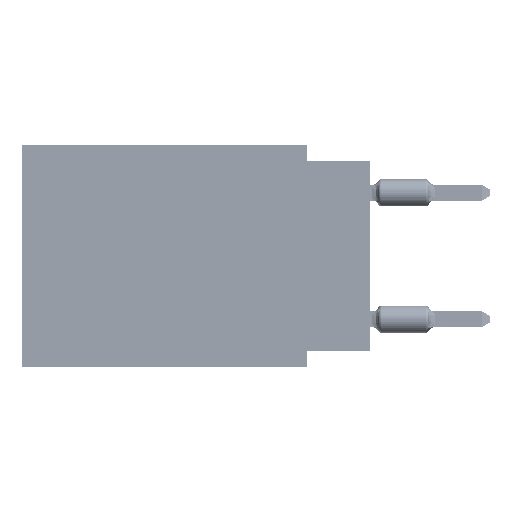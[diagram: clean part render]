
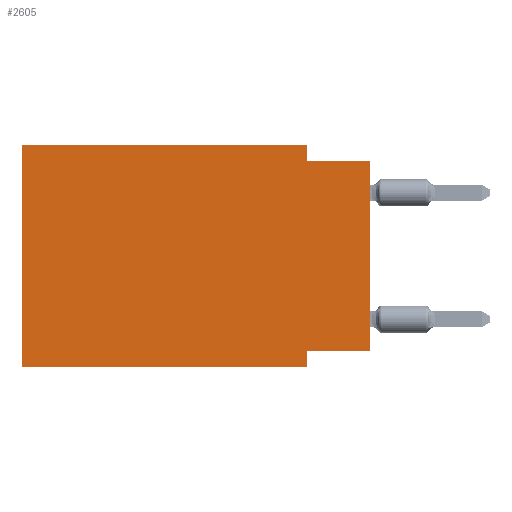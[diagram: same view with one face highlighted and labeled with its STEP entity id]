
A CAD part, left-side view. The second image highlights one B-rep face of the part: STEP entity #2605.
In plain terms, the highlighted planar face has unit normal (-1, 0, 0).
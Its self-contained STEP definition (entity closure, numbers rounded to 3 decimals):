
#426 = LINE ( 'NONE', #57246, #10804 ) ;
#1411 = ORIENTED_EDGE ( 'NONE', *, *, #46097, .F. ) ;
#2605 = ADVANCED_FACE ( 'NONE', ( #30433 ), #25722, .F. ) ;
#3043 = EDGE_CURVE ( 'NONE', #26202, #23078, #17483, .T. ) ;
#6856 = EDGE_CURVE ( 'NONE', #44678, #13129, #14527, .T. ) ;
#10655 = LINE ( 'NONE', #24699, #14334 ) ;
#10804 = VECTOR ( 'NONE', #43178, 1000. ) ;
#12487 = DIRECTION ( 'NONE',  ( 0., -1., 0. ) ) ;
#12929 = LINE ( 'NONE', #26066, #41188 ) ;
#13129 = VERTEX_POINT ( 'NONE', #49657 ) ;
#14241 = CARTESIAN_POINT ( 'NONE',  ( 0., 2.54, -0.635 ) ) ;
#14334 = VECTOR ( 'NONE', #34679, 1000. ) ;
#14527 = LINE ( 'NONE', #56056, #20309 ) ;
#17483 = LINE ( 'NONE', #32137, #44723 ) ;
#18924 = CARTESIAN_POINT ( 'NONE',  ( 0., 13.97, 0. ) ) ;
#20309 = VECTOR ( 'NONE', #41982, 1000. ) ;
#20555 = CARTESIAN_POINT ( 'NONE',  ( 0., 2.54, -8.89 ) ) ;
#22082 = VECTOR ( 'NONE', #31061, 1000. ) ;
#23078 = VERTEX_POINT ( 'NONE', #20555 ) ;
#23688 = EDGE_CURVE ( 'NONE', #13129, #52349, #59477, .T. ) ;
#24699 = CARTESIAN_POINT ( 'NONE',  ( 0., 0., 0. ) ) ;
#24920 = CARTESIAN_POINT ( 'NONE',  ( 0., 13.97, 0. ) ) ;
#25722 = PLANE ( 'NONE',  #50125 ) ;
#26066 = CARTESIAN_POINT ( 'NONE',  ( 0., 2.54, -8.89 ) ) ;
#26202 = VERTEX_POINT ( 'NONE', #37062 ) ;
#27254 = VECTOR ( 'NONE', #61697, 1000. ) ;
#28068 = LINE ( 'NONE', #52106, #59864 ) ;
#28915 = LINE ( 'NONE', #18924, #27254 ) ;
#29995 = EDGE_CURVE ( 'NONE', #55369, #46451, #10655, .T. ) ;
#30433 = FACE_OUTER_BOUND ( 'NONE', #59432, .T. ) ;
#31061 = DIRECTION ( 'NONE',  ( 0., 0., -1. ) ) ;
#32137 = CARTESIAN_POINT ( 'NONE',  ( 0., 13.97, -8.89 ) ) ;
#32706 = ORIENTED_EDGE ( 'NONE', *, *, #44882, .F. ) ;
#32989 = VERTEX_POINT ( 'NONE', #52696 ) ;
#34679 = DIRECTION ( 'NONE',  ( 0., 0., 1. ) ) ;
#35048 = CARTESIAN_POINT ( 'NONE',  ( 0., 0., -8.255 ) ) ;
#35105 = DIRECTION ( 'NONE',  ( 0., 0., -1. ) ) ;
#37062 = CARTESIAN_POINT ( 'NONE',  ( 0., 13.97, -8.89 ) ) ;
#37529 = ORIENTED_EDGE ( 'NONE', *, *, #6856, .F. ) ;
#37694 = ORIENTED_EDGE ( 'NONE', *, *, #55129, .F. ) ;
#40541 = ORIENTED_EDGE ( 'NONE', *, *, #23688, .F. ) ;
#41188 = VECTOR ( 'NONE', #45103, 1000. ) ;
#41982 = DIRECTION ( 'NONE',  ( 0., -1., 0. ) ) ;
#42424 = DIRECTION ( 'NONE',  ( 0., -1., 0. ) ) ;
#43178 = DIRECTION ( 'NONE',  ( 0., 1., 0. ) ) ;
#43928 = EDGE_CURVE ( 'NONE', #32989, #23078, #12929, .T. ) ;
#44156 = ORIENTED_EDGE ( 'NONE', *, *, #29995, .T. ) ;
#44678 = VERTEX_POINT ( 'NONE', #24920 ) ;
#44723 = VECTOR ( 'NONE', #12487, 1000. ) ;
#44882 = EDGE_CURVE ( 'NONE', #26202, #44678, #28915, .T. ) ;
#45103 = DIRECTION ( 'NONE',  ( 0., 0., -1. ) ) ;
#46097 = EDGE_CURVE ( 'NONE', #52349, #46451, #28068, .T. ) ;
#46451 = VERTEX_POINT ( 'NONE', #47879 ) ;
#47879 = CARTESIAN_POINT ( 'NONE',  ( 0., 0., -0.635 ) ) ;
#49154 = CARTESIAN_POINT ( 'NONE',  ( 0., 13.97, 0. ) ) ;
#49657 = CARTESIAN_POINT ( 'NONE',  ( 0., 2.54, 0. ) ) ;
#50125 = AXIS2_PLACEMENT_3D ( 'NONE', #49154, #54450, #35105 ) ;
#50896 = ORIENTED_EDGE ( 'NONE', *, *, #3043, .T. ) ;
#51017 = CARTESIAN_POINT ( 'NONE',  ( 0., 2.54, 0. ) ) ;
#52106 = CARTESIAN_POINT ( 'NONE',  ( 0., 0., -0.635 ) ) ;
#52349 = VERTEX_POINT ( 'NONE', #14241 ) ;
#52696 = CARTESIAN_POINT ( 'NONE',  ( 0., 2.54, -8.255 ) ) ;
#54450 = DIRECTION ( 'NONE',  ( 1., 0., 0. ) ) ;
#55129 = EDGE_CURVE ( 'NONE', #55369, #32989, #426, .T. ) ;
#55369 = VERTEX_POINT ( 'NONE', #35048 ) ;
#55822 = ORIENTED_EDGE ( 'NONE', *, *, #43928, .F. ) ;
#56056 = CARTESIAN_POINT ( 'NONE',  ( 0., 13.97, 0. ) ) ;
#57246 = CARTESIAN_POINT ( 'NONE',  ( 0., 0., -8.255 ) ) ;
#59432 = EDGE_LOOP ( 'NONE', ( #44156, #1411, #40541, #37529, #32706, #50896, #55822, #37694 ) ) ;
#59477 = LINE ( 'NONE', #51017, #22082 ) ;
#59864 = VECTOR ( 'NONE', #42424, 1000. ) ;
#61697 = DIRECTION ( 'NONE',  ( 0., 0., 1. ) ) ;
